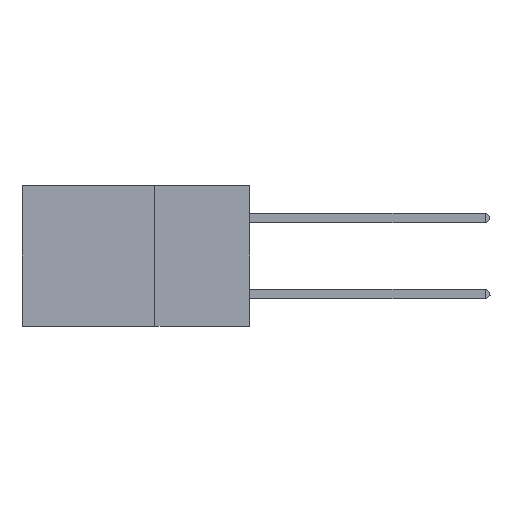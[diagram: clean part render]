
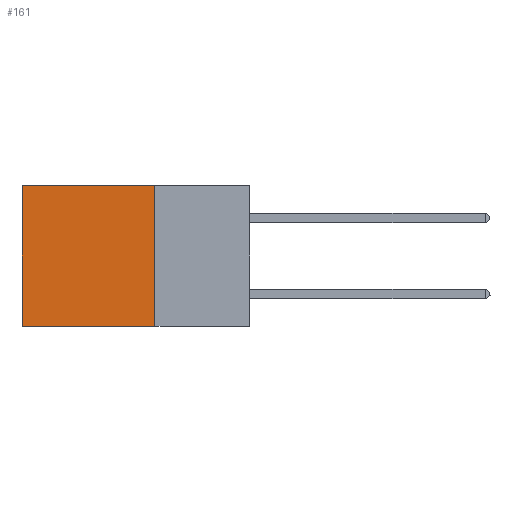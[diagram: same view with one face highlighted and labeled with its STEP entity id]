
A CAD part, left-side view. The second image highlights one B-rep face of the part: STEP entity #161.
In plain terms, the highlighted planar face has unit normal (-1, 0, 0).
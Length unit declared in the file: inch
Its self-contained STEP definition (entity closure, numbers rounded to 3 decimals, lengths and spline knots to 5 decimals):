
#161 = ADVANCED_FACE ( 'NONE', ( #1507 ), #2730, .F. ) ;
#726 = EDGE_CURVE ( 'NONE', #17283, #12055, #7375, .T. ) ;
#1324 = VERTEX_POINT ( 'NONE', #15496 ) ;
#1507 = FACE_OUTER_BOUND ( 'NONE', #3682, .T. ) ;
#1616 = ORIENTED_EDGE ( 'NONE', *, *, #17709, .T. ) ;
#1678 = CARTESIAN_POINT ( 'NONE',  ( 0.2875, 0.6, 0. ) ) ;
#2148 = LINE ( 'NONE', #18792, #5675 ) ;
#2302 = LINE ( 'NONE', #12212, #10293 ) ;
#2730 = PLANE ( 'NONE',  #4797 ) ;
#3682 = EDGE_LOOP ( 'NONE', ( #1616, #10666, #5808, #18606 ) ) ;
#4049 = CARTESIAN_POINT ( 'NONE',  ( 0.2875, 0.6, 0. ) ) ;
#4797 = AXIS2_PLACEMENT_3D ( 'NONE', #5871, #7131, #13275 ) ;
#5256 = EDGE_CURVE ( 'NONE', #17283, #1324, #2302, .T. ) ;
#5675 = VECTOR ( 'NONE', #8526, 39.37008 ) ;
#5808 = ORIENTED_EDGE ( 'NONE', *, *, #5256, .F. ) ;
#5871 = CARTESIAN_POINT ( 'NONE',  ( 0.2875, 0.25, 0. ) ) ;
#6895 = VECTOR ( 'NONE', #16647, 39.37008 ) ;
#7131 = DIRECTION ( 'NONE',  ( 1., 0., 0. ) ) ;
#7304 = CARTESIAN_POINT ( 'NONE',  ( 0.2875, 0.25, 0. ) ) ;
#7375 = LINE ( 'NONE', #13697, #6895 ) ;
#8334 = EDGE_CURVE ( 'NONE', #1324, #12040, #2148, .T. ) ;
#8526 = DIRECTION ( 'NONE',  ( 0., 1., 0. ) ) ;
#8842 = DIRECTION ( 'NONE',  ( 0., 0., -1. ) ) ;
#8952 = VECTOR ( 'NONE', #17508, 39.37008 ) ;
#10293 = VECTOR ( 'NONE', #8842, 39.37008 ) ;
#10666 = ORIENTED_EDGE ( 'NONE', *, *, #8334, .F. ) ;
#12040 = VERTEX_POINT ( 'NONE', #12336 ) ;
#12055 = VERTEX_POINT ( 'NONE', #1678 ) ;
#12212 = CARTESIAN_POINT ( 'NONE',  ( 0.2875, 0.25, 0. ) ) ;
#12336 = CARTESIAN_POINT ( 'NONE',  ( 0.2875, 0.6, -0.37 ) ) ;
#13275 = DIRECTION ( 'NONE',  ( 0., 0., -1. ) ) ;
#13697 = CARTESIAN_POINT ( 'NONE',  ( 0.2875, 0.25, 0. ) ) ;
#14262 = LINE ( 'NONE', #4049, #8952 ) ;
#15496 = CARTESIAN_POINT ( 'NONE',  ( 0.2875, 0.25, -0.37 ) ) ;
#16647 = DIRECTION ( 'NONE',  ( 0., 1., 0. ) ) ;
#17283 = VERTEX_POINT ( 'NONE', #7304 ) ;
#17508 = DIRECTION ( 'NONE',  ( 0., 0., -1. ) ) ;
#17709 = EDGE_CURVE ( 'NONE', #12055, #12040, #14262, .T. ) ;
#18606 = ORIENTED_EDGE ( 'NONE', *, *, #726, .T. ) ;
#18792 = CARTESIAN_POINT ( 'NONE',  ( 0.2875, 0.25, -0.37 ) ) ;
